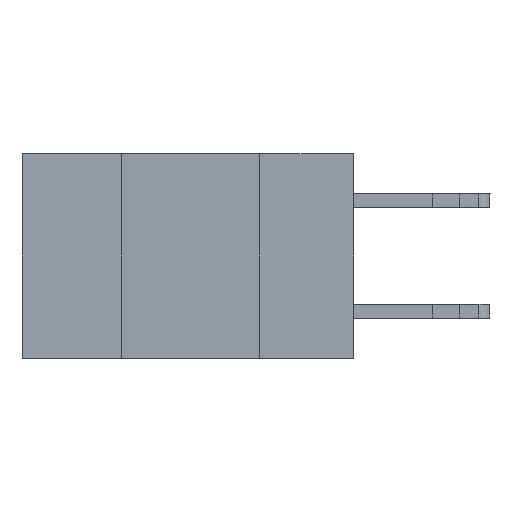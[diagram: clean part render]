
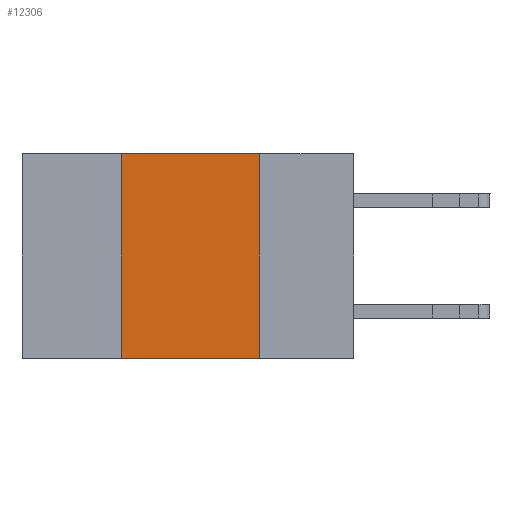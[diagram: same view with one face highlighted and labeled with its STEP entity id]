
A CAD part, left-side view. The second image highlights one B-rep face of the part: STEP entity #12306.
In plain terms, the highlighted planar face has unit normal (-1, 0, 0).
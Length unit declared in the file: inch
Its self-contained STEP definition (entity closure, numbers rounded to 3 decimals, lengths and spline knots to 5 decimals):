
#711 = EDGE_CURVE ( 'NONE', #20363, #19928, #3453, .T. ) ;
#1713 = CARTESIAN_POINT ( 'NONE',  ( 0., 0.6, -0.37 ) ) ;
#1889 = VERTEX_POINT ( 'NONE', #16772 ) ;
#2550 = LINE ( 'NONE', #25898, #6242 ) ;
#2668 = CARTESIAN_POINT ( 'NONE',  ( 0., 0.6, 0. ) ) ;
#3160 = CARTESIAN_POINT ( 'NONE',  ( 0., 0.42, 0. ) ) ;
#3453 = LINE ( 'NONE', #1713, #24203 ) ;
#5203 = CARTESIAN_POINT ( 'NONE',  ( 0., 0.6, 0. ) ) ;
#5324 = DIRECTION ( 'NONE',  ( 0., -1., 0. ) ) ;
#6242 = VECTOR ( 'NONE', #17542, 39.37008 ) ;
#12306 = ADVANCED_FACE ( 'NONE', ( #31721 ), #28733, .F. ) ;
#13336 = DIRECTION ( 'NONE',  ( 0., -1., 0. ) ) ;
#14076 = ORIENTED_EDGE ( 'NONE', *, *, #711, .T. ) ;
#16772 = CARTESIAN_POINT ( 'NONE',  ( 0., 0.42, 0. ) ) ;
#16810 = VECTOR ( 'NONE', #13336, 39.37008 ) ;
#17542 = DIRECTION ( 'NONE',  ( 0., 0., -1. ) ) ;
#17746 = AXIS2_PLACEMENT_3D ( 'NONE', #5203, #26417, #34075 ) ;
#17861 = CARTESIAN_POINT ( 'NONE',  ( 0., 0.17, 0. ) ) ;
#18411 = VERTEX_POINT ( 'NONE', #17861 ) ;
#18891 = CARTESIAN_POINT ( 'NONE',  ( 0., 0.42, -0.37 ) ) ;
#19928 = VERTEX_POINT ( 'NONE', #28926 ) ;
#20078 = DIRECTION ( 'NONE',  ( 0., 0., 1. ) ) ;
#20363 = VERTEX_POINT ( 'NONE', #18891 ) ;
#21160 = ORIENTED_EDGE ( 'NONE', *, *, #24299, .F. ) ;
#24203 = VECTOR ( 'NONE', #5324, 39.37008 ) ;
#24299 = EDGE_CURVE ( 'NONE', #18411, #19928, #2550, .T. ) ;
#24302 = LINE ( 'NONE', #3160, #27633 ) ;
#24303 = EDGE_LOOP ( 'NONE', ( #21160, #28392, #27823, #14076 ) ) ;
#25898 = CARTESIAN_POINT ( 'NONE',  ( 0., 0.17, 0. ) ) ;
#25945 = LINE ( 'NONE', #2668, #16810 ) ;
#26417 = DIRECTION ( 'NONE',  ( 1., 0., 0. ) ) ;
#27614 = EDGE_CURVE ( 'NONE', #20363, #1889, #24302, .T. ) ;
#27633 = VECTOR ( 'NONE', #20078, 39.37008 ) ;
#27823 = ORIENTED_EDGE ( 'NONE', *, *, #27614, .F. ) ;
#28067 = EDGE_CURVE ( 'NONE', #1889, #18411, #25945, .T. ) ;
#28392 = ORIENTED_EDGE ( 'NONE', *, *, #28067, .F. ) ;
#28733 = PLANE ( 'NONE',  #17746 ) ;
#28926 = CARTESIAN_POINT ( 'NONE',  ( 0., 0.17, -0.37 ) ) ;
#31721 = FACE_OUTER_BOUND ( 'NONE', #24303, .T. ) ;
#34075 = DIRECTION ( 'NONE',  ( 0., 0., -1. ) ) ;
